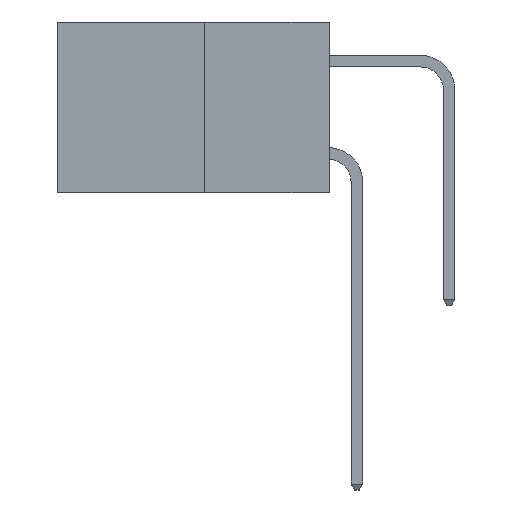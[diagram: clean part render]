
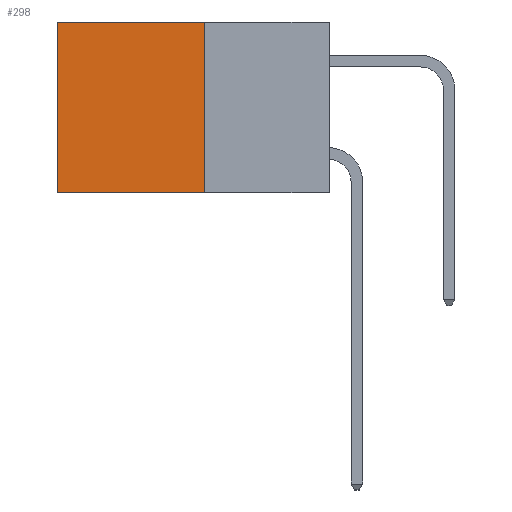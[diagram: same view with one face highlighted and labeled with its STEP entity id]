
A CAD part, left-side view. The second image highlights one B-rep face of the part: STEP entity #298.
In plain terms, the highlighted planar face has unit normal (-1, 0, 0).
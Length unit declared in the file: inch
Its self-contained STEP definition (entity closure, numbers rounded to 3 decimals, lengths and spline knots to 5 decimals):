
#13 = CARTESIAN_POINT ( 'NONE',  ( 0.277, 0.27, 0. ) ) ;
#298 = ADVANCED_FACE ( 'NONE', ( #2631 ), #2922, .F. ) ;
#554 = DIRECTION ( 'NONE',  ( 0., 0., -1. ) ) ;
#586 = VERTEX_POINT ( 'NONE', #7105 ) ;
#780 = VECTOR ( 'NONE', #9765, 39.37008 ) ;
#1450 = VECTOR ( 'NONE', #1699, 39.37008 ) ;
#1699 = DIRECTION ( 'NONE',  ( 0., 1., 0. ) ) ;
#2191 = VERTEX_POINT ( 'NONE', #13 ) ;
#2505 = DIRECTION ( 'NONE',  ( 1., 0., 0. ) ) ;
#2631 = FACE_OUTER_BOUND ( 'NONE', #10682, .T. ) ;
#2828 = ORIENTED_EDGE ( 'NONE', *, *, #3290, .T. ) ;
#2922 = PLANE ( 'NONE',  #7944 ) ;
#3024 = EDGE_CURVE ( 'NONE', #2191, #5117, #6599, .T. ) ;
#3290 = EDGE_CURVE ( 'NONE', #2191, #7472, #3926, .T. ) ;
#3615 = CARTESIAN_POINT ( 'NONE',  ( 0.277, 0.27, -0.37 ) ) ;
#3926 = LINE ( 'NONE', #12773, #1450 ) ;
#5117 = VERTEX_POINT ( 'NONE', #9739 ) ;
#5306 = ORIENTED_EDGE ( 'NONE', *, *, #8734, .F. ) ;
#5929 = VECTOR ( 'NONE', #12546, 39.37008 ) ;
#6399 = EDGE_CURVE ( 'NONE', #7472, #586, #7077, .T. ) ;
#6599 = LINE ( 'NONE', #3615, #780 ) ;
#7077 = LINE ( 'NONE', #8418, #12538 ) ;
#7105 = CARTESIAN_POINT ( 'NONE',  ( 0.277, 0.59, -0.37 ) ) ;
#7472 = VERTEX_POINT ( 'NONE', #10053 ) ;
#7944 = AXIS2_PLACEMENT_3D ( 'NONE', #9146, #2505, #554 ) ;
#8418 = CARTESIAN_POINT ( 'NONE',  ( 0.277, 0.59, -0.37 ) ) ;
#8613 = LINE ( 'NONE', #12806, #5929 ) ;
#8734 = EDGE_CURVE ( 'NONE', #5117, #586, #8613, .T. ) ;
#9146 = CARTESIAN_POINT ( 'NONE',  ( 0.277, 0.27, -0.37 ) ) ;
#9739 = CARTESIAN_POINT ( 'NONE',  ( 0.277, 0.27, -0.37 ) ) ;
#9765 = DIRECTION ( 'NONE',  ( 0., 0., -1. ) ) ;
#10053 = CARTESIAN_POINT ( 'NONE',  ( 0.277, 0.59, 0. ) ) ;
#10682 = EDGE_LOOP ( 'NONE', ( #13094, #5306, #10783, #2828 ) ) ;
#10783 = ORIENTED_EDGE ( 'NONE', *, *, #3024, .F. ) ;
#11799 = DIRECTION ( 'NONE',  ( 0., 0., -1. ) ) ;
#12538 = VECTOR ( 'NONE', #11799, 39.37008 ) ;
#12546 = DIRECTION ( 'NONE',  ( 0., 1., 0. ) ) ;
#12773 = CARTESIAN_POINT ( 'NONE',  ( 0.277, 0.27, 0. ) ) ;
#12806 = CARTESIAN_POINT ( 'NONE',  ( 0.277, 0.27, -0.37 ) ) ;
#13094 = ORIENTED_EDGE ( 'NONE', *, *, #6399, .T. ) ;
